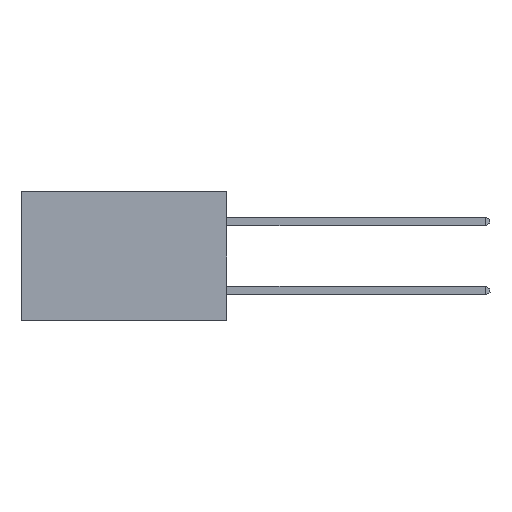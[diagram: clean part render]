
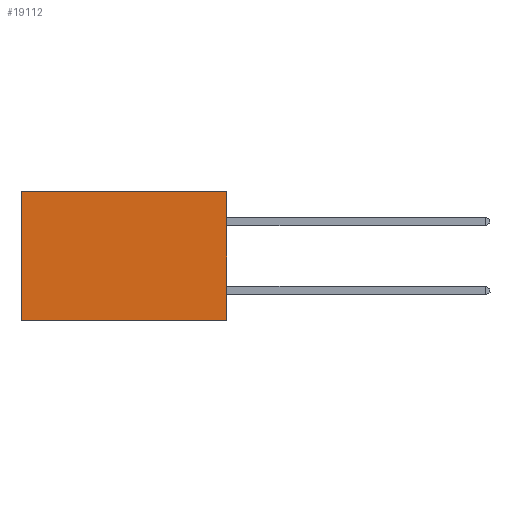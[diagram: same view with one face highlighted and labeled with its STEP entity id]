
A CAD part, left-side view. The second image highlights one B-rep face of the part: STEP entity #19112.
In plain terms, the highlighted planar face has unit normal (-1, 0, 0).
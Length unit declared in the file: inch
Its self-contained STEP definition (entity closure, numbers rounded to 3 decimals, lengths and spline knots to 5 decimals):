
#258 = ORIENTED_EDGE ( 'NONE', *, *, #12463, .T. ) ;
#825 = DIRECTION ( 'NONE',  ( 0., 1., 0. ) ) ;
#935 = AXIS2_PLACEMENT_3D ( 'NONE', #12727, #17996, #18117 ) ;
#2028 = LINE ( 'NONE', #11595, #16929 ) ;
#3572 = EDGE_CURVE ( 'NONE', #12345, #28516, #20262, .T. ) ;
#4210 = CARTESIAN_POINT ( 'NONE',  ( 0.277, 0., 0. ) ) ;
#6663 = CARTESIAN_POINT ( 'NONE',  ( 0.277, 0., -0.37 ) ) ;
#7541 = DIRECTION ( 'NONE',  ( 0., 0., -1. ) ) ;
#7562 = EDGE_CURVE ( 'NONE', #12345, #22093, #19142, .T. ) ;
#7633 = CARTESIAN_POINT ( 'NONE',  ( 0.277, 0., -0.37 ) ) ;
#8730 = ORIENTED_EDGE ( 'NONE', *, *, #7562, .T. ) ;
#9486 = LINE ( 'NONE', #27647, #15752 ) ;
#11595 = CARTESIAN_POINT ( 'NONE',  ( 0.277, 0., -0.37 ) ) ;
#12345 = VERTEX_POINT ( 'NONE', #26870 ) ;
#12463 = EDGE_CURVE ( 'NONE', #22093, #13716, #9486, .T. ) ;
#12727 = CARTESIAN_POINT ( 'NONE',  ( 0.277, 0., -0.37 ) ) ;
#13716 = VERTEX_POINT ( 'NONE', #27028 ) ;
#14503 = DIRECTION ( 'NONE',  ( 0., 0., -1. ) ) ;
#14825 = EDGE_LOOP ( 'NONE', ( #258, #26547, #32715, #8730 ) ) ;
#15449 = PLANE ( 'NONE',  #935 ) ;
#15752 = VECTOR ( 'NONE', #14503, 39.37008 ) ;
#16929 = VECTOR ( 'NONE', #27473, 39.37008 ) ;
#17805 = CARTESIAN_POINT ( 'NONE',  ( 0.277, 0.59, 0. ) ) ;
#17996 = DIRECTION ( 'NONE',  ( 1., 0., 0. ) ) ;
#18117 = DIRECTION ( 'NONE',  ( 0., 0., -1. ) ) ;
#18614 = VECTOR ( 'NONE', #7541, 39.37008 ) ;
#19112 = ADVANCED_FACE ( 'NONE', ( #30125 ), #15449, .F. ) ;
#19142 = LINE ( 'NONE', #4210, #26156 ) ;
#20262 = LINE ( 'NONE', #6663, #18614 ) ;
#22093 = VERTEX_POINT ( 'NONE', #17805 ) ;
#24698 = EDGE_CURVE ( 'NONE', #28516, #13716, #2028, .T. ) ;
#26156 = VECTOR ( 'NONE', #825, 39.37008 ) ;
#26547 = ORIENTED_EDGE ( 'NONE', *, *, #24698, .F. ) ;
#26870 = CARTESIAN_POINT ( 'NONE',  ( 0.277, 0., 0. ) ) ;
#27028 = CARTESIAN_POINT ( 'NONE',  ( 0.277, 0.59, -0.37 ) ) ;
#27473 = DIRECTION ( 'NONE',  ( 0., 1., 0. ) ) ;
#27647 = CARTESIAN_POINT ( 'NONE',  ( 0.277, 0.59, -0.37 ) ) ;
#28516 = VERTEX_POINT ( 'NONE', #7633 ) ;
#30125 = FACE_OUTER_BOUND ( 'NONE', #14825, .T. ) ;
#32715 = ORIENTED_EDGE ( 'NONE', *, *, #3572, .F. ) ;
